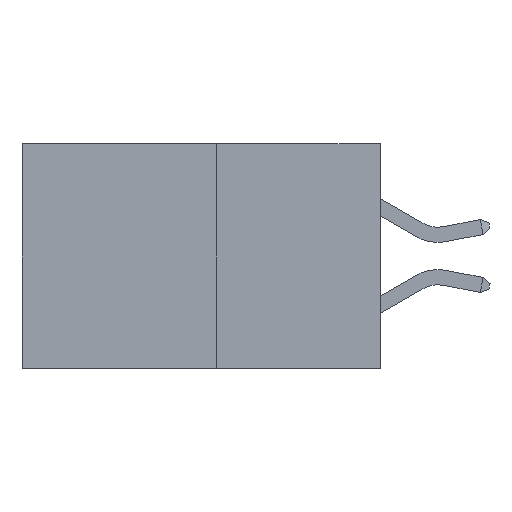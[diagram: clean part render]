
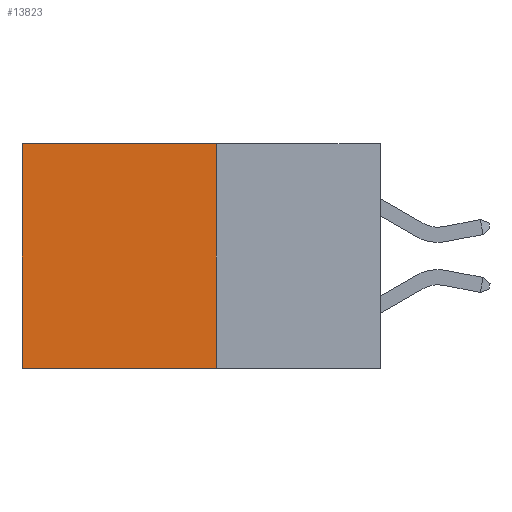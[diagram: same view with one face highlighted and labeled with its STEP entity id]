
A CAD part, left-side view. The second image highlights one B-rep face of the part: STEP entity #13823.
In plain terms, the highlighted planar face has unit normal (-1, 0, 0).
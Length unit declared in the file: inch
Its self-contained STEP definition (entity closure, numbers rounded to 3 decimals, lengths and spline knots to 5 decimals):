
#827 = ORIENTED_EDGE ( 'NONE', *, *, #12752, .T. ) ;
#1522 = CARTESIAN_POINT ( 'NONE',  ( 0.277, 0.27, 0. ) ) ;
#2550 = FACE_OUTER_BOUND ( 'NONE', #4566, .T. ) ;
#4243 = VECTOR ( 'NONE', #34691, 39.37008 ) ;
#4335 = DIRECTION ( 'NONE',  ( 0., 0., -1. ) ) ;
#4451 = CARTESIAN_POINT ( 'NONE',  ( 0.277, 0.59, -0.37 ) ) ;
#4566 = EDGE_LOOP ( 'NONE', ( #8511, #6222, #19413, #827 ) ) ;
#5044 = DIRECTION ( 'NONE',  ( 0., 0., -1. ) ) ;
#5086 = DIRECTION ( 'NONE',  ( 1., 0., 0. ) ) ;
#5294 = PLANE ( 'NONE',  #5873 ) ;
#5367 = CARTESIAN_POINT ( 'NONE',  ( 0.277, 0.27, -0.37 ) ) ;
#5746 = LINE ( 'NONE', #18021, #26776 ) ;
#5873 = AXIS2_PLACEMENT_3D ( 'NONE', #5367, #5086, #5044 ) ;
#6222 = ORIENTED_EDGE ( 'NONE', *, *, #19539, .F. ) ;
#8511 = ORIENTED_EDGE ( 'NONE', *, *, #13867, .T. ) ;
#8772 = VERTEX_POINT ( 'NONE', #1522 ) ;
#9057 = VERTEX_POINT ( 'NONE', #29783 ) ;
#11954 = VERTEX_POINT ( 'NONE', #34050 ) ;
#12752 = EDGE_CURVE ( 'NONE', #8772, #9057, #21571, .T. ) ;
#13823 = ADVANCED_FACE ( 'NONE', ( #2550 ), #5294, .F. ) ;
#13867 = EDGE_CURVE ( 'NONE', #9057, #11954, #17171, .T. ) ;
#17171 = LINE ( 'NONE', #4451, #22756 ) ;
#18021 = CARTESIAN_POINT ( 'NONE',  ( 0.277, 0.27, -0.37 ) ) ;
#19413 = ORIENTED_EDGE ( 'NONE', *, *, #25094, .F. ) ;
#19539 = EDGE_CURVE ( 'NONE', #23194, #11954, #5746, .T. ) ;
#21571 = LINE ( 'NONE', #21842, #35139 ) ;
#21721 = DIRECTION ( 'NONE',  ( 0., 1., 0. ) ) ;
#21842 = CARTESIAN_POINT ( 'NONE',  ( 0.277, 0.27, 0. ) ) ;
#22756 = VECTOR ( 'NONE', #4335, 39.37008 ) ;
#23194 = VERTEX_POINT ( 'NONE', #35326 ) ;
#25094 = EDGE_CURVE ( 'NONE', #8772, #23194, #26167, .T. ) ;
#26167 = LINE ( 'NONE', #31968, #4243 ) ;
#26776 = VECTOR ( 'NONE', #34357, 39.37008 ) ;
#29783 = CARTESIAN_POINT ( 'NONE',  ( 0.277, 0.59, 0. ) ) ;
#31968 = CARTESIAN_POINT ( 'NONE',  ( 0.277, 0.27, -0.37 ) ) ;
#34050 = CARTESIAN_POINT ( 'NONE',  ( 0.277, 0.59, -0.37 ) ) ;
#34357 = DIRECTION ( 'NONE',  ( 0., 1., 0. ) ) ;
#34691 = DIRECTION ( 'NONE',  ( 0., 0., -1. ) ) ;
#35139 = VECTOR ( 'NONE', #21721, 39.37008 ) ;
#35326 = CARTESIAN_POINT ( 'NONE',  ( 0.277, 0.27, -0.37 ) ) ;
